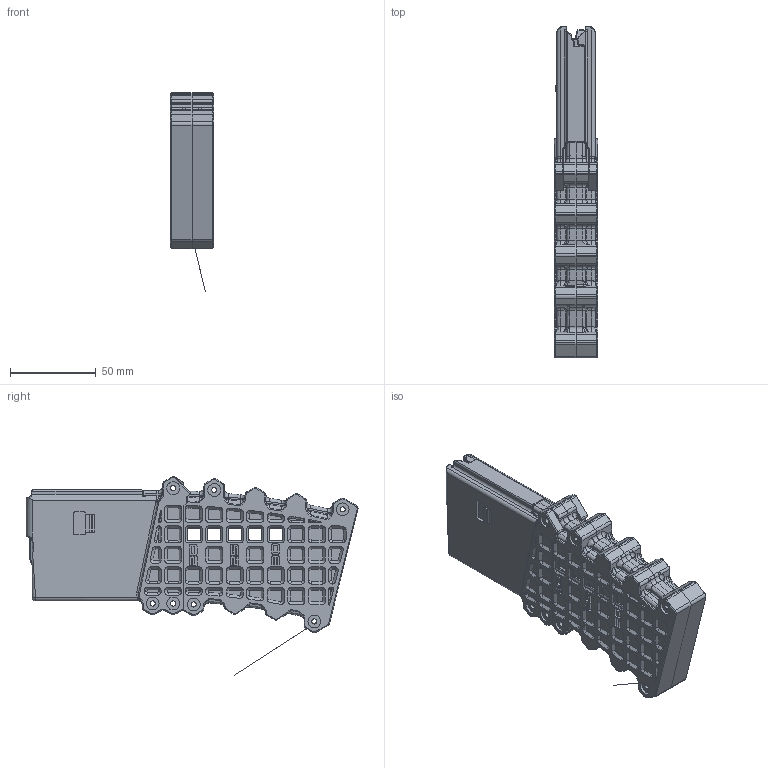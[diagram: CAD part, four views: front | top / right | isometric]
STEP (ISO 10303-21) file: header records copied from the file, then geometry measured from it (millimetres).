
FILE_DESCRIPTION (( 'STEP AP214' ), '1' );
FILE_NAME ('Waffle Windowed Magazine.STEP', '2021-05-01T22:59:00', ( '' ), ( '' ), 'SwSTEP 2.0', 'SolidWorks 2020', '' );
FILE_SCHEMA (( 'AUTOMOTIVE_DESIGN' ));
Length unit declared in the file: millimetre
Products named in the file (5): Mag Body Top; Mag Follower; Mag Body Bottom Left Windowed; Waffle Windowed Magazine; Mag Body Bottom Right Windowed
Assembly tree (4 placements, depth 2):
  Waffle Windowed Magazine
    Mag Body Top
    Mag Body Bottom Left Windowed
    Mag Body Bottom Right Windowed
    Mag Follower
Bounding box: 25.5 x 194 x 115.95 mm (x, y, z)
Volume: 115737.3 mm3; surface area: 83394.7 mm2
Topology: 4 solids, 6 shells, 3476 faces, 8990 edges, 5527 vertices
Faces by surface type: plane 1090, cylinder 877, bspline 812, cone 455, torus 212, sphere 30
Entity records: 134932 total; most frequent: CARTESIAN_POINT 56094, ORIENTED_EDGE 17738, DIRECTION 14825, EDGE_CURVE 8869, VERTEX_POINT 5519, AXIS2_PLACEMENT_3D 5384, LINE 4057, VECTOR 4057
